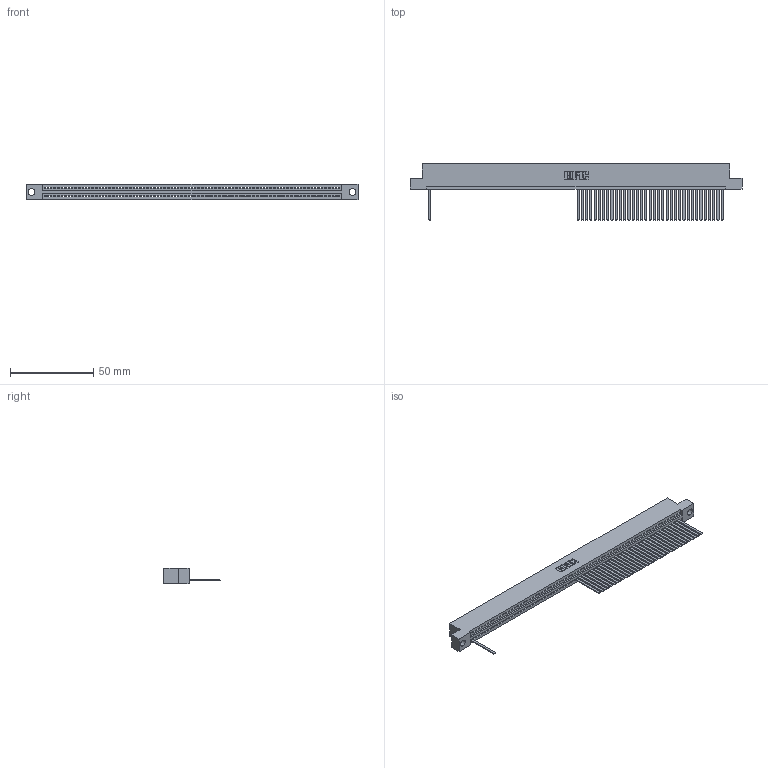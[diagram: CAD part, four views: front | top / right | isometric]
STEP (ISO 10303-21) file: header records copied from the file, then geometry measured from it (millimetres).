
FILE_DESCRIPTION (( 'STEP AP203' ), '1' );
FILE_NAME ('395-070-544-104.STEP', '2018-11-26T22:35:07', ( '' ), ( '' ), 'SwSTEP 2.0', 'SolidWorks 2016', '' );
FILE_SCHEMA (( 'CONFIG_CONTROL_DESIGN' ));
Length unit declared in the file: inch
Products named in the file (3): 345-292-001_345-293-144; 345 Part_Flush Mounting Lugs - 0.156 Dia-TH; 395-070-544-104
Assembly tree (37 placements, depth 2):
  395-070-544-104
    345 Part_Flush Mounting Lugs - 0.156 Dia-TH
    345-292-001_345-293-144  x36
Bounding box: 199.01 x 33.96 x 9.4 mm (x, y, z)
Volume: 19071.2 mm3; surface area: 24717.3 mm2
Topology: 37 solids, 37 shells, 2542 faces, 7865 edges, 5194 vertices
Faces by surface type: plane 1852, cylinder 690
Entity records: 47645 total; most frequent: ORIENTED_EDGE 8450, CARTESIAN_POINT 8412, DIRECTION 7265, EDGE_CURVE 4225, VECTOR 3817, LINE 3817, VERTEX_POINT 2814, AXIS2_PLACEMENT_3D 1724
